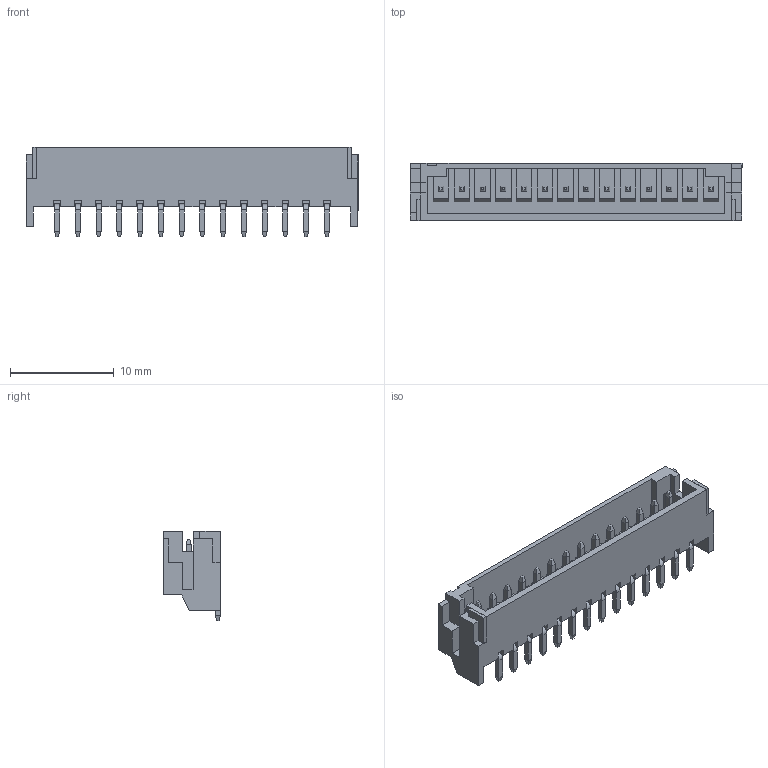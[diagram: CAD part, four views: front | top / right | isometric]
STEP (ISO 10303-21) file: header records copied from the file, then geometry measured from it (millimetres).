
FILE_DESCRIPTION (( 'STEP AP203' ), '1' );
FILE_NAME ('140-514-417-060.STEP', '2020-03-31T20:25:35', ( '' ), ( '' ), 'SwSTEP 2.0', 'SolidWorks 2016', '' );
FILE_SCHEMA (( 'CONFIG_CONTROL_DESIGN' ));
Length unit declared in the file: millimetre
Products named in the file (4): RA SMT Contact; RA SMT Pad; RA SMT Housing_514; 140-514-417-060
Assembly tree (17 placements, depth 2):
  140-514-417-060
    RA SMT Housing_514
    RA SMT Contact  x14
    RA SMT Pad  x2
Bounding box: 32 x 5.5 x 8.65 mm (x, y, z)
Volume: 420.4 mm3; surface area: 1608.1 mm2
Topology: 17 solids, 17 shells, 724 faces, 1744 edges, 1050 vertices
Faces by surface type: plane 668, cylinder 56
Entity records: 11482 total; most frequent: CARTESIAN_POINT 1926, ORIENTED_EDGE 1904, DIRECTION 1656, EDGE_CURVE 952, LINE 944, VECTOR 944, VERTEX_POINT 626, EDGE_LOOP 356
